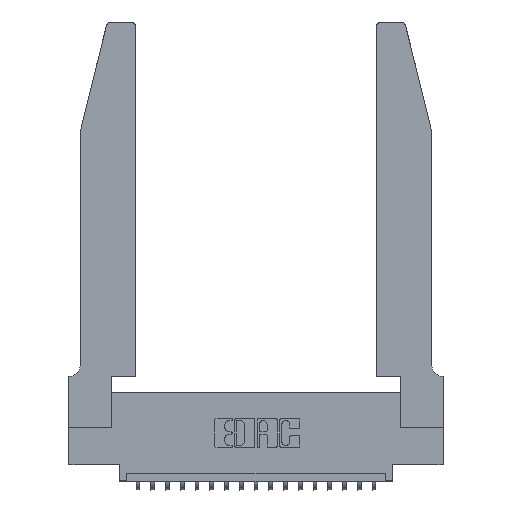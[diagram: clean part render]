
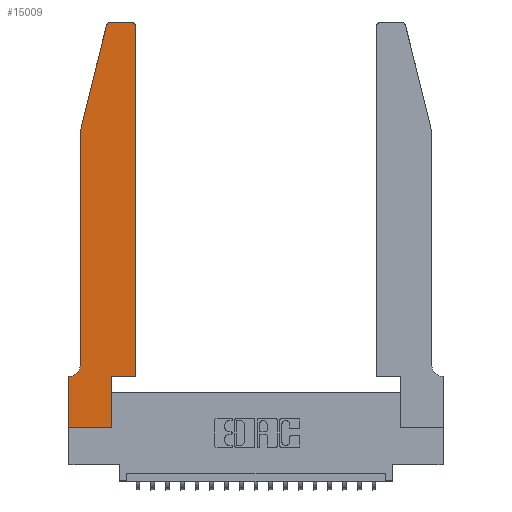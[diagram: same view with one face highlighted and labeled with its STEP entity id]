
A CAD part, top view. The second image highlights one B-rep face of the part: STEP entity #15009.
In plain terms, the highlighted planar face has unit normal (0, 0, 1).
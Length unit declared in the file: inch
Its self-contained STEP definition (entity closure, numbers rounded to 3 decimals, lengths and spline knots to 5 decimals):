
#35 = DIRECTION ( 'NONE',  ( 0., 1., 0. ) ) ;
#181 = CARTESIAN_POINT ( 'NONE',  ( 0., 0.35, 0.37 ) ) ;
#358 = DIRECTION ( 'NONE',  ( 1., 0., 0. ) ) ;
#426 = DIRECTION ( 'NONE',  ( 0., 0., 1. ) ) ;
#520 = CARTESIAN_POINT ( 'NONE',  ( 0., 0.35, 0.37 ) ) ;
#681 = VERTEX_POINT ( 'NONE', #6812 ) ;
#741 = DIRECTION ( 'NONE',  ( -1., 0., 0. ) ) ;
#759 = DIRECTION ( 'NONE',  ( 1., 0., 0. ) ) ;
#812 = DIRECTION ( 'NONE',  ( 0., 0., -1. ) ) ;
#820 = LINE ( 'NONE', #6944, #13363 ) ;
#1224 = ORIENTED_EDGE ( 'NONE', *, *, #2819, .T. ) ;
#1253 = VECTOR ( 'NONE', #759, 39.37008 ) ;
#1357 = EDGE_CURVE ( 'NONE', #6163, #10987, #14284, .T. ) ;
#1768 = ORIENTED_EDGE ( 'NONE', *, *, #20922, .T. ) ;
#2457 = LINE ( 'NONE', #16707, #9616 ) ;
#2504 = DIRECTION ( 'NONE',  ( 0., -1., 0. ) ) ;
#2509 = VERTEX_POINT ( 'NONE', #4704 ) ;
#2609 = VERTEX_POINT ( 'NONE', #6673 ) ;
#2819 = EDGE_CURVE ( 'NONE', #20145, #19800, #19546, .T. ) ;
#2947 = LINE ( 'NONE', #20511, #19788 ) ;
#3243 = VECTOR ( 'NONE', #741, 39.37008 ) ;
#3355 = CARTESIAN_POINT ( 'NONE',  ( 0.2865, 0.35, 0.37 ) ) ;
#3794 = ORIENTED_EDGE ( 'NONE', *, *, #11736, .T. ) ;
#4136 = CIRCLE ( 'NONE', #20100, 0.03 ) ;
#4463 = ORIENTED_EDGE ( 'NONE', *, *, #1357, .T. ) ;
#4600 = CARTESIAN_POINT ( 'NONE',  ( 0.0755, 2., 0.37 ) ) ;
#4704 = CARTESIAN_POINT ( 'NONE',  ( 0.0755, 0.42, 0.37 ) ) ;
#5052 = DIRECTION ( 'NONE',  ( 0., -1., 0. ) ) ;
#5388 = ORIENTED_EDGE ( 'NONE', *, *, #13768, .T. ) ;
#5454 = DIRECTION ( 'NONE',  ( 0., 0., 1. ) ) ;
#5662 = CARTESIAN_POINT ( 'NONE',  ( 0.0055, 0.42, 0.37 ) ) ;
#5803 = ORIENTED_EDGE ( 'NONE', *, *, #21052, .T. ) ;
#6163 = VERTEX_POINT ( 'NONE', #10066 ) ;
#6673 = CARTESIAN_POINT ( 'NONE',  ( 0.2865, 0.35, 0.37 ) ) ;
#6812 = CARTESIAN_POINT ( 'NONE',  ( 0.25487, 2.72718, 0.37 ) ) ;
#6944 = CARTESIAN_POINT ( 'NONE',  ( 0.2605, 2.75, 0.37 ) ) ;
#6986 = ORIENTED_EDGE ( 'NONE', *, *, #7626, .T. ) ;
#7390 = VERTEX_POINT ( 'NONE', #7996 ) ;
#7626 = EDGE_CURVE ( 'NONE', #681, #8609, #2947, .T. ) ;
#7814 = AXIS2_PLACEMENT_3D ( 'NONE', #5662, #812, #10525 ) ;
#7996 = CARTESIAN_POINT ( 'NONE',  ( 0.4505, 0.35, 0.37 ) ) ;
#8009 = LINE ( 'NONE', #19275, #19487 ) ;
#8609 = VERTEX_POINT ( 'NONE', #4600 ) ;
#8750 = LINE ( 'NONE', #20231, #15397 ) ;
#8936 = CARTESIAN_POINT ( 'NONE',  ( 0.0755, 0.35, 0.37 ) ) ;
#9023 = EDGE_LOOP ( 'NONE', ( #1768, #5803, #6986, #17300, #16235, #1224, #5388, #4463, #3794, #12819, #18671, #11023 ) ) ;
#9029 = VERTEX_POINT ( 'NONE', #17663 ) ;
#9183 = VECTOR ( 'NONE', #35, 39.37008 ) ;
#9616 = VECTOR ( 'NONE', #5052, 39.37008 ) ;
#9713 = LINE ( 'NONE', #3355, #9183 ) ;
#9762 = PLANE ( 'NONE',  #12293 ) ;
#9833 = EDGE_CURVE ( 'NONE', #7390, #9029, #8750, .T. ) ;
#10066 = CARTESIAN_POINT ( 'NONE',  ( 0., 0., 0.37 ) ) ;
#10525 = DIRECTION ( 'NONE',  ( -1., 0., 0. ) ) ;
#10853 = VERTEX_POINT ( 'NONE', #18330 ) ;
#10952 = AXIS2_PLACEMENT_3D ( 'NONE', #20029, #426, #358 ) ;
#10987 = VERTEX_POINT ( 'NONE', #12373 ) ;
#11023 = ORIENTED_EDGE ( 'NONE', *, *, #18655, .T. ) ;
#11210 = VERTEX_POINT ( 'NONE', #18316 ) ;
#11241 = CARTESIAN_POINT ( 'NONE',  ( 0.0055, 0.35, 0.37 ) ) ;
#11736 = EDGE_CURVE ( 'NONE', #10987, #2609, #9713, .T. ) ;
#11961 = DIRECTION ( 'NONE',  ( 1., 0., 0. ) ) ;
#12293 = AXIS2_PLACEMENT_3D ( 'NONE', #181, #13281, #16322 ) ;
#12373 = CARTESIAN_POINT ( 'NONE',  ( 0.2865, 0., 0.37 ) ) ;
#12819 = ORIENTED_EDGE ( 'NONE', *, *, #19674, .T. ) ;
#13281 = DIRECTION ( 'NONE',  ( 0., 0., 1. ) ) ;
#13363 = VECTOR ( 'NONE', #18129, 39.37008 ) ;
#13768 = EDGE_CURVE ( 'NONE', #19800, #6163, #2457, .T. ) ;
#13796 = DIRECTION ( 'NONE',  ( 1., 0., 0. ) ) ;
#14284 = LINE ( 'NONE', #16794, #1253 ) ;
#15009 = ADVANCED_FACE ( 'NONE', ( #17704 ), #9762, .T. ) ;
#15397 = VECTOR ( 'NONE', #20163, 39.37008 ) ;
#15718 = CIRCLE ( 'NONE', #10952, 0.03 ) ;
#16235 = ORIENTED_EDGE ( 'NONE', *, *, #19885, .T. ) ;
#16322 = DIRECTION ( 'NONE',  ( 1., 0., 0. ) ) ;
#16611 = VECTOR ( 'NONE', #2504, 39.37008 ) ;
#16707 = CARTESIAN_POINT ( 'NONE',  ( 0., 0., 0.37 ) ) ;
#16794 = CARTESIAN_POINT ( 'NONE',  ( 0., 0., 0.37 ) ) ;
#16922 = CIRCLE ( 'NONE', #7814, 0.07 ) ;
#17110 = CARTESIAN_POINT ( 'NONE',  ( 0.284, 2.72, 0.37 ) ) ;
#17300 = ORIENTED_EDGE ( 'NONE', *, *, #17764, .T. ) ;
#17663 = CARTESIAN_POINT ( 'NONE',  ( 0.4505, 2.72, 0.37 ) ) ;
#17704 = FACE_OUTER_BOUND ( 'NONE', #9023, .T. ) ;
#17764 = EDGE_CURVE ( 'NONE', #8609, #2509, #18864, .T. ) ;
#18129 = DIRECTION ( 'NONE',  ( -1., 0., 0. ) ) ;
#18316 = CARTESIAN_POINT ( 'NONE',  ( 0.4205, 2.75, 0.37 ) ) ;
#18330 = CARTESIAN_POINT ( 'NONE',  ( 0.284, 2.75, 0.37 ) ) ;
#18655 = EDGE_CURVE ( 'NONE', #9029, #11210, #15718, .T. ) ;
#18671 = ORIENTED_EDGE ( 'NONE', *, *, #9833, .T. ) ;
#18864 = LINE ( 'NONE', #20454, #16611 ) ;
#18935 = DIRECTION ( 'NONE',  ( -0.239, -0.971, 0. ) ) ;
#19275 = CARTESIAN_POINT ( 'NONE',  ( 0.4505, 0.35, 0.37 ) ) ;
#19487 = VECTOR ( 'NONE', #11961, 39.37008 ) ;
#19546 = LINE ( 'NONE', #8936, #3243 ) ;
#19674 = EDGE_CURVE ( 'NONE', #2609, #7390, #8009, .T. ) ;
#19788 = VECTOR ( 'NONE', #18935, 39.37008 ) ;
#19800 = VERTEX_POINT ( 'NONE', #520 ) ;
#19885 = EDGE_CURVE ( 'NONE', #2509, #20145, #16922, .T. ) ;
#20029 = CARTESIAN_POINT ( 'NONE',  ( 0.4205, 2.72, 0.37 ) ) ;
#20100 = AXIS2_PLACEMENT_3D ( 'NONE', #17110, #5454, #13796 ) ;
#20145 = VERTEX_POINT ( 'NONE', #11241 ) ;
#20163 = DIRECTION ( 'NONE',  ( 0., 1., 0. ) ) ;
#20231 = CARTESIAN_POINT ( 'NONE',  ( 0.4505, 0.35, 0.37 ) ) ;
#20454 = CARTESIAN_POINT ( 'NONE',  ( 0.0755, 2., 0.37 ) ) ;
#20511 = CARTESIAN_POINT ( 'NONE',  ( 0.0755, 2., 0.37 ) ) ;
#20922 = EDGE_CURVE ( 'NONE', #11210, #10853, #820, .T. ) ;
#21052 = EDGE_CURVE ( 'NONE', #10853, #681, #4136, .T. ) ;
